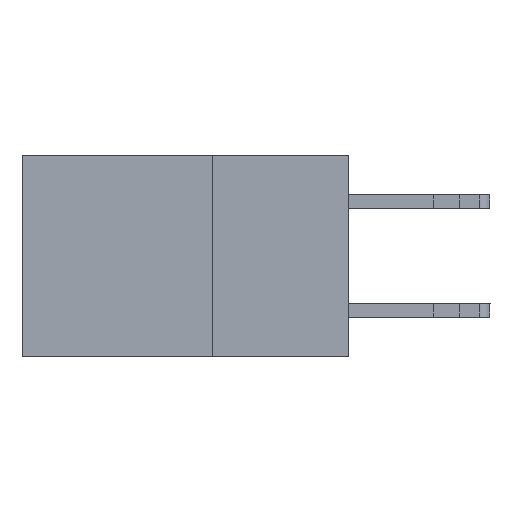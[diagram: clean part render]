
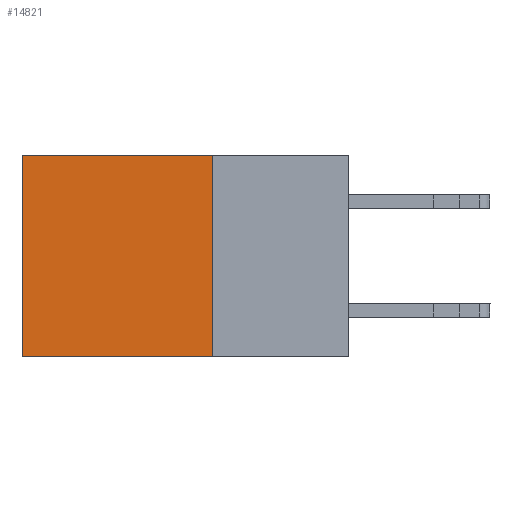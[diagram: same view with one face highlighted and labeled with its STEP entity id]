
A CAD part, left-side view. The second image highlights one B-rep face of the part: STEP entity #14821.
In plain terms, the highlighted planar face has unit normal (-1, 0, 0).
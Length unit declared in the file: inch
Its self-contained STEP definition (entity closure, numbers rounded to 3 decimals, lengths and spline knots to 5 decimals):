
#468 = VECTOR ( 'NONE', #11697, 39.37008 ) ;
#671 = PLANE ( 'NONE',  #13819 ) ;
#870 = DIRECTION ( 'NONE',  ( 0., 0., -1. ) ) ;
#2392 = EDGE_CURVE ( 'NONE', #10469, #3655, #13615, .T. ) ;
#2914 = CARTESIAN_POINT ( 'NONE',  ( 0.298, 0.25, 0. ) ) ;
#2990 = EDGE_CURVE ( 'NONE', #10469, #5544, #16765, .T. ) ;
#3224 = ORIENTED_EDGE ( 'NONE', *, *, #2990, .T. ) ;
#3655 = VERTEX_POINT ( 'NONE', #5654 ) ;
#4334 = LINE ( 'NONE', #8102, #10075 ) ;
#4739 = CARTESIAN_POINT ( 'NONE',  ( 0.298, 0.25, 0. ) ) ;
#5544 = VERTEX_POINT ( 'NONE', #13338 ) ;
#5553 = DIRECTION ( 'NONE',  ( 0., 1., 0. ) ) ;
#5654 = CARTESIAN_POINT ( 'NONE',  ( 0.298, 0.25, -0.37 ) ) ;
#6247 = DIRECTION ( 'NONE',  ( 0., 1., 0. ) ) ;
#6560 = EDGE_CURVE ( 'NONE', #3655, #8778, #4334, .T. ) ;
#7206 = CARTESIAN_POINT ( 'NONE',  ( 0.298, 0.25, 0. ) ) ;
#7492 = ORIENTED_EDGE ( 'NONE', *, *, #6560, .F. ) ;
#8096 = ORIENTED_EDGE ( 'NONE', *, *, #11751, .T. ) ;
#8102 = CARTESIAN_POINT ( 'NONE',  ( 0.298, 0.25, -0.37 ) ) ;
#8778 = VERTEX_POINT ( 'NONE', #17310 ) ;
#10075 = VECTOR ( 'NONE', #5553, 39.37008 ) ;
#10205 = CARTESIAN_POINT ( 'NONE',  ( 0.298, 0.6, 0. ) ) ;
#10469 = VERTEX_POINT ( 'NONE', #2914 ) ;
#11129 = LINE ( 'NONE', #10205, #11358 ) ;
#11358 = VECTOR ( 'NONE', #870, 39.37008 ) ;
#11697 = DIRECTION ( 'NONE',  ( 0., 0., -1. ) ) ;
#11751 = EDGE_CURVE ( 'NONE', #5544, #8778, #11129, .T. ) ;
#12211 = ORIENTED_EDGE ( 'NONE', *, *, #2392, .F. ) ;
#13338 = CARTESIAN_POINT ( 'NONE',  ( 0.298, 0.6, 0. ) ) ;
#13584 = VECTOR ( 'NONE', #6247, 39.37008 ) ;
#13615 = LINE ( 'NONE', #15848, #468 ) ;
#13819 = AXIS2_PLACEMENT_3D ( 'NONE', #4739, #14149, #15485 ) ;
#13850 = FACE_OUTER_BOUND ( 'NONE', #14350, .T. ) ;
#14149 = DIRECTION ( 'NONE',  ( 1., 0., 0. ) ) ;
#14350 = EDGE_LOOP ( 'NONE', ( #8096, #7492, #12211, #3224 ) ) ;
#14821 = ADVANCED_FACE ( 'NONE', ( #13850 ), #671, .F. ) ;
#15485 = DIRECTION ( 'NONE',  ( 0., 0., -1. ) ) ;
#15848 = CARTESIAN_POINT ( 'NONE',  ( 0.298, 0.25, 0. ) ) ;
#16765 = LINE ( 'NONE', #7206, #13584 ) ;
#17310 = CARTESIAN_POINT ( 'NONE',  ( 0.298, 0.6, -0.37 ) ) ;
